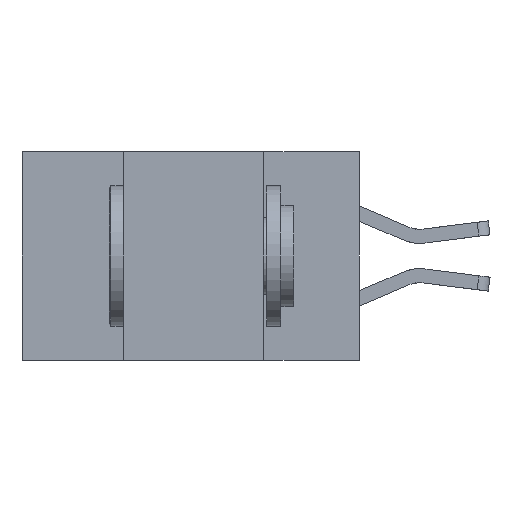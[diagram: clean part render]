
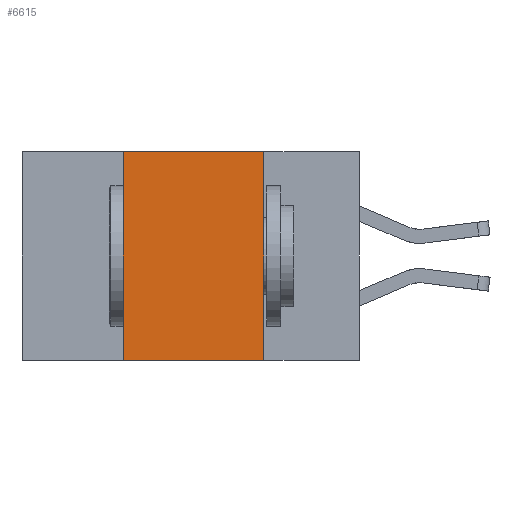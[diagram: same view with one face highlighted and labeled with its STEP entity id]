
A CAD part, left-side view. The second image highlights one B-rep face of the part: STEP entity #6615.
In plain terms, the highlighted planar face has unit normal (-1, 0, 0).
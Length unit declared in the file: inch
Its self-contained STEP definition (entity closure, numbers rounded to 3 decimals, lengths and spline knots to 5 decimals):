
#402 = ORIENTED_EDGE ( 'NONE', *, *, #12357, .F. ) ;
#923 = EDGE_LOOP ( 'NONE', ( #10212, #402, #13830, #10326 ) ) ;
#1159 = CARTESIAN_POINT ( 'NONE',  ( 0., 0.6, 0. ) ) ;
#1513 = CARTESIAN_POINT ( 'NONE',  ( 0., 0.6, 0. ) ) ;
#1585 = DIRECTION ( 'NONE',  ( 0., -1., 0. ) ) ;
#2100 = EDGE_CURVE ( 'NONE', #10129, #13994, #6681, .T. ) ;
#2310 = VERTEX_POINT ( 'NONE', #6342 ) ;
#2682 = DIRECTION ( 'NONE',  ( 0., -1., 0. ) ) ;
#3049 = LINE ( 'NONE', #5780, #3242 ) ;
#3242 = VECTOR ( 'NONE', #7361, 39.37008 ) ;
#3875 = LINE ( 'NONE', #7447, #13851 ) ;
#5703 = CARTESIAN_POINT ( 'NONE',  ( 0., 0.17, -0.37 ) ) ;
#5780 = CARTESIAN_POINT ( 'NONE',  ( 0., 0.42, 0. ) ) ;
#6342 = CARTESIAN_POINT ( 'NONE',  ( 0., 0.42, 0. ) ) ;
#6615 = ADVANCED_FACE ( 'NONE', ( #12249 ), #13985, .F. ) ;
#6681 = LINE ( 'NONE', #9584, #8348 ) ;
#7361 = DIRECTION ( 'NONE',  ( 0., 0., 1. ) ) ;
#7447 = CARTESIAN_POINT ( 'NONE',  ( 0., 0.6, -0.37 ) ) ;
#7860 = CARTESIAN_POINT ( 'NONE',  ( 0., 0.42, -0.37 ) ) ;
#8348 = VECTOR ( 'NONE', #14315, 39.37008 ) ;
#9584 = CARTESIAN_POINT ( 'NONE',  ( 0., 0.17, 0. ) ) ;
#9788 = EDGE_CURVE ( 'NONE', #10010, #13994, #3875, .T. ) ;
#10010 = VERTEX_POINT ( 'NONE', #7860 ) ;
#10129 = VERTEX_POINT ( 'NONE', #13705 ) ;
#10212 = ORIENTED_EDGE ( 'NONE', *, *, #2100, .F. ) ;
#10326 = ORIENTED_EDGE ( 'NONE', *, *, #9788, .T. ) ;
#11742 = DIRECTION ( 'NONE',  ( 1., 0., 0. ) ) ;
#12215 = AXIS2_PLACEMENT_3D ( 'NONE', #1159, #11742, #14035 ) ;
#12249 = FACE_OUTER_BOUND ( 'NONE', #923, .T. ) ;
#12357 = EDGE_CURVE ( 'NONE', #2310, #10129, #14854, .T. ) ;
#12560 = EDGE_CURVE ( 'NONE', #10010, #2310, #3049, .T. ) ;
#13592 = VECTOR ( 'NONE', #2682, 39.37008 ) ;
#13705 = CARTESIAN_POINT ( 'NONE',  ( 0., 0.17, 0. ) ) ;
#13830 = ORIENTED_EDGE ( 'NONE', *, *, #12560, .F. ) ;
#13851 = VECTOR ( 'NONE', #1585, 39.37008 ) ;
#13985 = PLANE ( 'NONE',  #12215 ) ;
#13994 = VERTEX_POINT ( 'NONE', #5703 ) ;
#14035 = DIRECTION ( 'NONE',  ( 0., 0., -1. ) ) ;
#14315 = DIRECTION ( 'NONE',  ( 0., 0., -1. ) ) ;
#14854 = LINE ( 'NONE', #1513, #13592 ) ;
